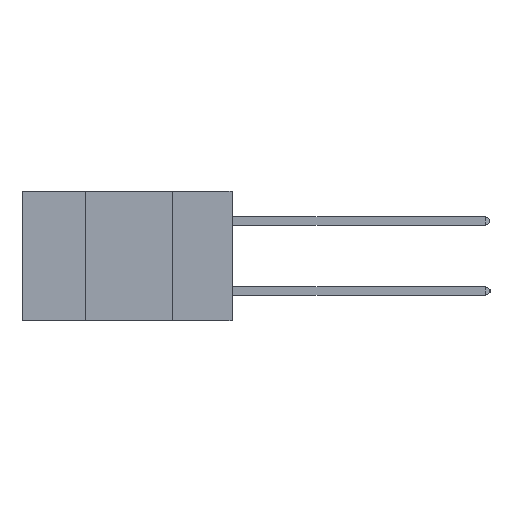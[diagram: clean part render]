
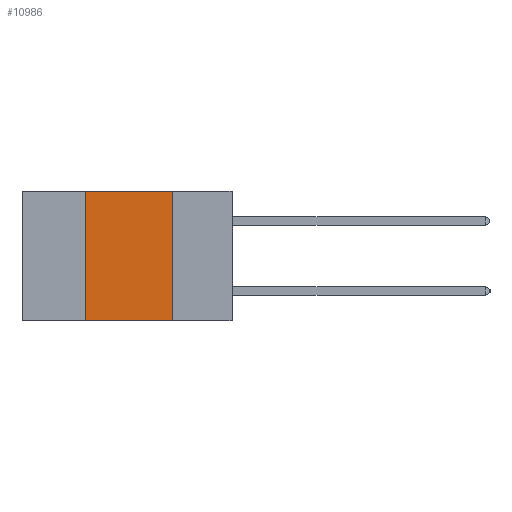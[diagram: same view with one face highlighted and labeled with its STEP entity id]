
A CAD part, left-side view. The second image highlights one B-rep face of the part: STEP entity #10986.
In plain terms, the highlighted planar face has unit normal (-1, 0, 0).
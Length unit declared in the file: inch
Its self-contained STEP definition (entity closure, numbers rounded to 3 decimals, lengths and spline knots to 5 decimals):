
#52 = VECTOR ( 'NONE', #11065, 39.37008 ) ;
#181 = EDGE_CURVE ( 'NONE', #1770, #8298, #6546, .T. ) ;
#210 = EDGE_CURVE ( 'NONE', #2986, #7688, #4012, .T. ) ;
#230 = EDGE_CURVE ( 'NONE', #2986, #1770, #3420, .T. ) ;
#271 = EDGE_CURVE ( 'NONE', #8298, #7688, #10264, .T. ) ;
#636 = CARTESIAN_POINT ( 'NONE',  ( 0., 0.42, -0.37 ) ) ;
#1440 = VECTOR ( 'NONE', #6049, 39.37008 ) ;
#1770 = VERTEX_POINT ( 'NONE', #6529 ) ;
#2658 = DIRECTION ( 'NONE',  ( 0., 0., 1. ) ) ;
#2986 = VERTEX_POINT ( 'NONE', #636 ) ;
#3404 = AXIS2_PLACEMENT_3D ( 'NONE', #9230, #5508, #11952 ) ;
#3420 = LINE ( 'NONE', #7218, #10559 ) ;
#3613 = PLANE ( 'NONE',  #3404 ) ;
#3841 = CARTESIAN_POINT ( 'NONE',  ( 0., 0.17, 0. ) ) ;
#3880 = ORIENTED_EDGE ( 'NONE', *, *, #210, .T. ) ;
#4012 = LINE ( 'NONE', #12222, #8704 ) ;
#5205 = ORIENTED_EDGE ( 'NONE', *, *, #271, .F. ) ;
#5508 = DIRECTION ( 'NONE',  ( 1., 0., 0. ) ) ;
#5812 = ORIENTED_EDGE ( 'NONE', *, *, #230, .F. ) ;
#6049 = DIRECTION ( 'NONE',  ( 0., -1., 0. ) ) ;
#6529 = CARTESIAN_POINT ( 'NONE',  ( 0., 0.42, 0. ) ) ;
#6546 = LINE ( 'NONE', #11901, #1440 ) ;
#6671 = CARTESIAN_POINT ( 'NONE',  ( 0., 0.17, 0. ) ) ;
#7218 = CARTESIAN_POINT ( 'NONE',  ( 0., 0.42, 0. ) ) ;
#7688 = VERTEX_POINT ( 'NONE', #10455 ) ;
#7992 = ORIENTED_EDGE ( 'NONE', *, *, #181, .F. ) ;
#8029 = FACE_OUTER_BOUND ( 'NONE', #8384, .T. ) ;
#8298 = VERTEX_POINT ( 'NONE', #6671 ) ;
#8384 = EDGE_LOOP ( 'NONE', ( #5205, #7992, #5812, #3880 ) ) ;
#8704 = VECTOR ( 'NONE', #9876, 39.37008 ) ;
#9230 = CARTESIAN_POINT ( 'NONE',  ( 0., 0.6, 0. ) ) ;
#9876 = DIRECTION ( 'NONE',  ( 0., -1., 0. ) ) ;
#10264 = LINE ( 'NONE', #3841, #52 ) ;
#10455 = CARTESIAN_POINT ( 'NONE',  ( 0., 0.17, -0.37 ) ) ;
#10559 = VECTOR ( 'NONE', #2658, 39.37008 ) ;
#10986 = ADVANCED_FACE ( 'NONE', ( #8029 ), #3613, .F. ) ;
#11065 = DIRECTION ( 'NONE',  ( 0., 0., -1. ) ) ;
#11901 = CARTESIAN_POINT ( 'NONE',  ( 0., 0.6, 0. ) ) ;
#11952 = DIRECTION ( 'NONE',  ( 0., 0., -1. ) ) ;
#12222 = CARTESIAN_POINT ( 'NONE',  ( 0., 0.6, -0.37 ) ) ;
